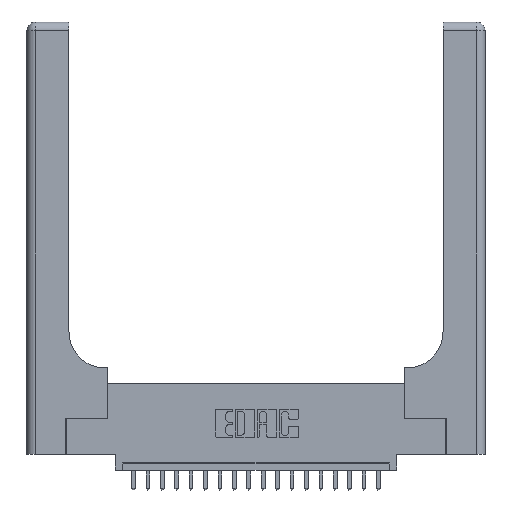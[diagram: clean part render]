
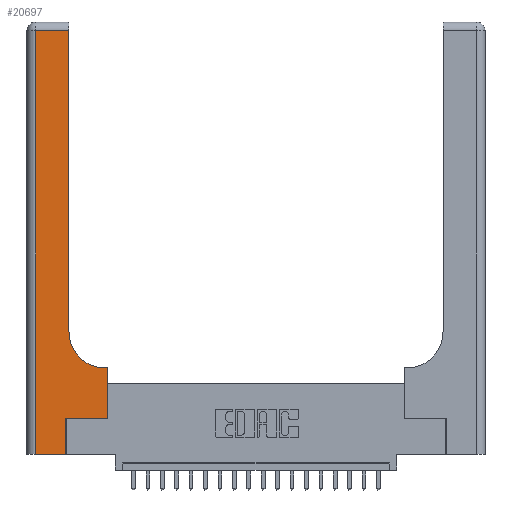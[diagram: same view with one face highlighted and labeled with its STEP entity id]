
A CAD part, top view. The second image highlights one B-rep face of the part: STEP entity #20697.
In plain terms, the highlighted planar face has unit normal (0, 0, 1).
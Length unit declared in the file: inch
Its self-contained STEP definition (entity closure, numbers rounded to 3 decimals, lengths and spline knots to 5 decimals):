
#650 = CARTESIAN_POINT ( 'NONE',  ( 0.269, 0.25, 0.37 ) ) ;
#890 = DIRECTION ( 'NONE',  ( -1., 0., 0. ) ) ;
#1561 = VECTOR ( 'NONE', #10164, 39.37008 ) ;
#1715 = LINE ( 'NONE', #6732, #6532 ) ;
#1913 = AXIS2_PLACEMENT_3D ( 'NONE', #19453, #9240, #21199 ) ;
#2250 = VECTOR ( 'NONE', #11905, 39.37008 ) ;
#2348 = EDGE_LOOP ( 'NONE', ( #3315, #18453, #3267, #13329, #11277, #4609, #11289, #8187, #14798 ) ) ;
#2467 = EDGE_CURVE ( 'NONE', #6165, #3279, #8383, .T. ) ;
#2943 = CARTESIAN_POINT ( 'NONE',  ( 0., 0., 0.37 ) ) ;
#3115 = DIRECTION ( 'NONE',  ( 0., 1., 0. ) ) ;
#3267 = ORIENTED_EDGE ( 'NONE', *, *, #3592, .T. ) ;
#3279 = VERTEX_POINT ( 'NONE', #17883 ) ;
#3315 = ORIENTED_EDGE ( 'NONE', *, *, #14455, .T. ) ;
#3494 = VECTOR ( 'NONE', #890, 39.37008 ) ;
#3521 = CARTESIAN_POINT ( 'NONE',  ( 0.269, 0.25, 0.37 ) ) ;
#3592 = EDGE_CURVE ( 'NONE', #20932, #18812, #1715, .T. ) ;
#4609 = ORIENTED_EDGE ( 'NONE', *, *, #2467, .T. ) ;
#4616 = VERTEX_POINT ( 'NONE', #17617 ) ;
#5155 = VERTEX_POINT ( 'NONE', #20444 ) ;
#5393 = DIRECTION ( 'NONE',  ( -1., 0., 0. ) ) ;
#6165 = VERTEX_POINT ( 'NONE', #3521 ) ;
#6532 = VECTOR ( 'NONE', #10152, 39.37008 ) ;
#6732 = CARTESIAN_POINT ( 'NONE',  ( 0.06, 3., 0.37 ) ) ;
#6761 = EDGE_CURVE ( 'NONE', #18812, #19710, #19608, .T. ) ;
#6779 = CARTESIAN_POINT ( 'NONE',  ( 0.269, 0., 0.37 ) ) ;
#8065 = DIRECTION ( 'NONE',  ( 1., 0., 0. ) ) ;
#8187 = ORIENTED_EDGE ( 'NONE', *, *, #9865, .T. ) ;
#8286 = CIRCLE ( 'NONE', #1913, 0.25 ) ;
#8383 = LINE ( 'NONE', #650, #15049 ) ;
#8485 = CARTESIAN_POINT ( 'NONE',  ( 0., 2.94, 0.37 ) ) ;
#9052 = CARTESIAN_POINT ( 'NONE',  ( 0.06, 2.94, 0.37 ) ) ;
#9240 = DIRECTION ( 'NONE',  ( 0., 0., -1. ) ) ;
#9865 = EDGE_CURVE ( 'NONE', #5155, #4616, #17075, .T. ) ;
#10152 = DIRECTION ( 'NONE',  ( 0., -1., 0. ) ) ;
#10164 = DIRECTION ( 'NONE',  ( 0., 1., 0. ) ) ;
#10423 = LINE ( 'NONE', #8485, #18206 ) ;
#11277 = ORIENTED_EDGE ( 'NONE', *, *, #13493, .T. ) ;
#11289 = ORIENTED_EDGE ( 'NONE', *, *, #17995, .T. ) ;
#11507 = CARTESIAN_POINT ( 'NONE',  ( 0.2915, 2.94, 0.37 ) ) ;
#11905 = DIRECTION ( 'NONE',  ( 0., 1., 0. ) ) ;
#12809 = CARTESIAN_POINT ( 'NONE',  ( 0.2915, 0.85, 0.37 ) ) ;
#13329 = ORIENTED_EDGE ( 'NONE', *, *, #6761, .T. ) ;
#13341 = AXIS2_PLACEMENT_3D ( 'NONE', #19120, #18983, #5393 ) ;
#13493 = EDGE_CURVE ( 'NONE', #19710, #6165, #15279, .T. ) ;
#13505 = CARTESIAN_POINT ( 'NONE',  ( 0.5585, 0.25, 0.37 ) ) ;
#13654 = PLANE ( 'NONE',  #13341 ) ;
#14214 = EDGE_CURVE ( 'NONE', #18373, #20932, #10423, .T. ) ;
#14455 = EDGE_CURVE ( 'NONE', #19233, #18373, #16336, .T. ) ;
#14541 = FACE_OUTER_BOUND ( 'NONE', #2348, .T. ) ;
#14798 = ORIENTED_EDGE ( 'NONE', *, *, #15982, .T. ) ;
#15049 = VECTOR ( 'NONE', #19170, 39.37008 ) ;
#15274 = CARTESIAN_POINT ( 'NONE',  ( 0.269, 0., 0.37 ) ) ;
#15279 = LINE ( 'NONE', #15274, #2250 ) ;
#15594 = VECTOR ( 'NONE', #8065, 39.37008 ) ;
#15982 = EDGE_CURVE ( 'NONE', #4616, #19233, #8286, .T. ) ;
#16142 = CARTESIAN_POINT ( 'NONE',  ( 0.2915, 0.6, 0.37 ) ) ;
#16336 = LINE ( 'NONE', #19183, #20584 ) ;
#16920 = DIRECTION ( 'NONE',  ( -1., 0., 0. ) ) ;
#17075 = LINE ( 'NONE', #16142, #3494 ) ;
#17617 = CARTESIAN_POINT ( 'NONE',  ( 0.5415, 0.6, 0.37 ) ) ;
#17883 = CARTESIAN_POINT ( 'NONE',  ( 0.5585, 0.25, 0.37 ) ) ;
#17995 = EDGE_CURVE ( 'NONE', #3279, #5155, #19659, .T. ) ;
#18206 = VECTOR ( 'NONE', #16920, 39.37008 ) ;
#18373 = VERTEX_POINT ( 'NONE', #11507 ) ;
#18453 = ORIENTED_EDGE ( 'NONE', *, *, #14214, .T. ) ;
#18812 = VERTEX_POINT ( 'NONE', #19088 ) ;
#18983 = DIRECTION ( 'NONE',  ( 0., 0., -1. ) ) ;
#19088 = CARTESIAN_POINT ( 'NONE',  ( 0.06, 0., 0.37 ) ) ;
#19120 = CARTESIAN_POINT ( 'NONE',  ( 0., 3., 0.37 ) ) ;
#19170 = DIRECTION ( 'NONE',  ( 1., 0., 0. ) ) ;
#19183 = CARTESIAN_POINT ( 'NONE',  ( 0.2915, 3., 0.37 ) ) ;
#19233 = VERTEX_POINT ( 'NONE', #12809 ) ;
#19453 = CARTESIAN_POINT ( 'NONE',  ( 0.5415, 0.85, 0.37 ) ) ;
#19608 = LINE ( 'NONE', #2943, #15594 ) ;
#19659 = LINE ( 'NONE', #13505, #1561 ) ;
#19710 = VERTEX_POINT ( 'NONE', #6779 ) ;
#20444 = CARTESIAN_POINT ( 'NONE',  ( 0.5585, 0.6, 0.37 ) ) ;
#20584 = VECTOR ( 'NONE', #3115, 39.37008 ) ;
#20697 = ADVANCED_FACE ( 'NONE', ( #14541 ), #13654, .F. ) ;
#20932 = VERTEX_POINT ( 'NONE', #9052 ) ;
#21199 = DIRECTION ( 'NONE',  ( 1., 0., 0. ) ) ;
